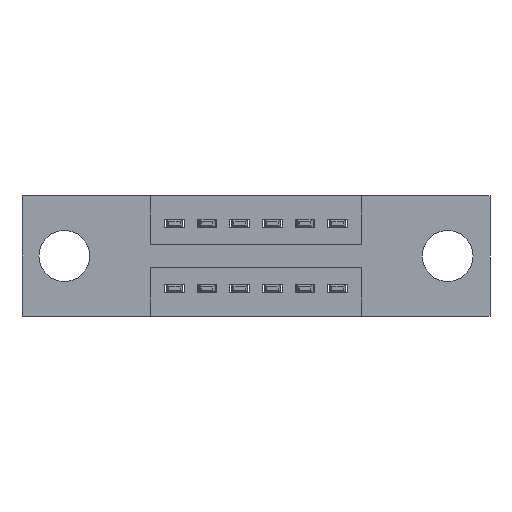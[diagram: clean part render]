
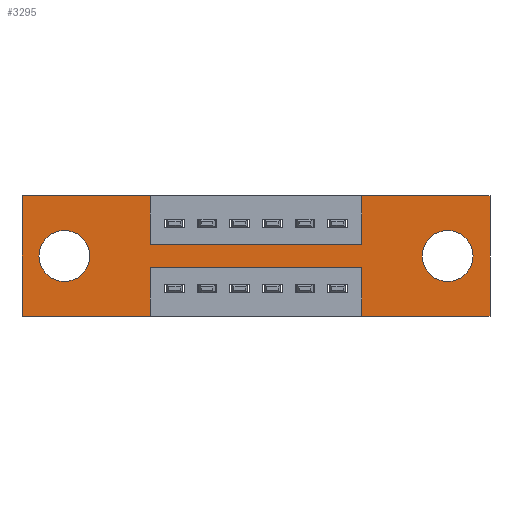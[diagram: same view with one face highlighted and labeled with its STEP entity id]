
A CAD part, front view. The second image highlights one B-rep face of the part: STEP entity #3295.
In plain terms, the highlighted planar face has unit normal (0, -1, 0).
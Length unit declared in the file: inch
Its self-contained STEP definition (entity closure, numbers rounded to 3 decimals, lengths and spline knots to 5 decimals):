
#187 = DIRECTION ( 'NONE',  ( -1., 0., 0. ) ) ;
#217 = VERTEX_POINT ( 'NONE', #2972 ) ;
#337 = LINE ( 'NONE', #4971, #4850 ) ;
#415 = EDGE_CURVE ( 'NONE', #9614, #4297, #8648, .T. ) ;
#434 = ORIENTED_EDGE ( 'NONE', *, *, #8055, .F. ) ;
#477 = CARTESIAN_POINT ( 'NONE',  ( 0.3925, 0., -0.37 ) ) ;
#515 = ORIENTED_EDGE ( 'NONE', *, *, #3587, .F. ) ;
#593 = DIRECTION ( 'NONE',  ( 0., 0., 1. ) ) ;
#698 = EDGE_CURVE ( 'NONE', #9111, #2674, #3773, .T. ) ;
#855 = DIRECTION ( 'NONE',  ( 0., 1., 0. ) ) ;
#882 = EDGE_CURVE ( 'NONE', #5985, #5519, #2591, .T. ) ;
#930 = CARTESIAN_POINT ( 'NONE',  ( 1.435, 0., -0.37 ) ) ;
#1006 = DIRECTION ( 'NONE',  ( 0., 1., 0. ) ) ;
#1039 = CARTESIAN_POINT ( 'NONE',  ( 1.0425, 0., -0.15 ) ) ;
#1098 = DIRECTION ( 'NONE',  ( 0., 0., 1. ) ) ;
#1200 = FACE_OUTER_BOUND ( 'NONE', #3306, .T. ) ;
#1219 = ORIENTED_EDGE ( 'NONE', *, *, #3712, .F. ) ;
#1236 = LINE ( 'NONE', #3494, #9543 ) ;
#1238 = DIRECTION ( 'NONE',  ( 0., 1., 0. ) ) ;
#1439 = EDGE_CURVE ( 'NONE', #4119, #7483, #1813, .T. ) ;
#1510 = CARTESIAN_POINT ( 'NONE',  ( 0., 0., 0. ) ) ;
#1564 = DIRECTION ( 'NONE',  ( -1., 0., 0. ) ) ;
#1686 = ORIENTED_EDGE ( 'NONE', *, *, #415, .T. ) ;
#1782 = VERTEX_POINT ( 'NONE', #6910 ) ;
#1813 = LINE ( 'NONE', #9343, #3753 ) ;
#1977 = VECTOR ( 'NONE', #4465, 39.37008 ) ;
#1980 = CARTESIAN_POINT ( 'NONE',  ( 0.13, 0., -0.185 ) ) ;
#2025 = LINE ( 'NONE', #477, #1977 ) ;
#2029 = DIRECTION ( 'NONE',  ( -1., 0., 0. ) ) ;
#2212 = LINE ( 'NONE', #5299, #7685 ) ;
#2216 = ORIENTED_EDGE ( 'NONE', *, *, #882, .F. ) ;
#2288 = CARTESIAN_POINT ( 'NONE',  ( 1.0425, 0., 0. ) ) ;
#2332 = CARTESIAN_POINT ( 'NONE',  ( 0.13, 0., -0.263 ) ) ;
#2591 = LINE ( 'NONE', #9475, #3455 ) ;
#2674 = VERTEX_POINT ( 'NONE', #2332 ) ;
#2708 = CARTESIAN_POINT ( 'NONE',  ( 1.305, 0., -0.107 ) ) ;
#2804 = AXIS2_PLACEMENT_3D ( 'NONE', #5584, #1006, #4055 ) ;
#2819 = ORIENTED_EDGE ( 'NONE', *, *, #8117, .T. ) ;
#2972 = CARTESIAN_POINT ( 'NONE',  ( 0.3925, 0., -0.22 ) ) ;
#3007 = DIRECTION ( 'NONE',  ( 0., 0., 1. ) ) ;
#3103 = LINE ( 'NONE', #6804, #7696 ) ;
#3113 = EDGE_CURVE ( 'NONE', #7722, #5985, #5393, .T. ) ;
#3295 = ADVANCED_FACE ( 'NONE', ( #8737, #4986, #1200 ), #3510, .T. ) ;
#3306 = EDGE_LOOP ( 'NONE', ( #434, #1219, #2216, #4464, #7397, #6076, #3683, #5480, #3716, #4623, #3730, #515 ) ) ;
#3455 = VECTOR ( 'NONE', #1098, 39.37008 ) ;
#3494 = CARTESIAN_POINT ( 'NONE',  ( 0., 0., 0. ) ) ;
#3510 = PLANE ( 'NONE',  #7396 ) ;
#3587 = EDGE_CURVE ( 'NONE', #8382, #5559, #3103, .T. ) ;
#3589 = EDGE_CURVE ( 'NONE', #7483, #3890, #8487, .T. ) ;
#3603 = VECTOR ( 'NONE', #6065, 39.37008 ) ;
#3683 = ORIENTED_EDGE ( 'NONE', *, *, #3589, .F. ) ;
#3712 = EDGE_CURVE ( 'NONE', #5519, #217, #337, .T. ) ;
#3716 = ORIENTED_EDGE ( 'NONE', *, *, #4641, .F. ) ;
#3730 = ORIENTED_EDGE ( 'NONE', *, *, #4853, .F. ) ;
#3753 = VECTOR ( 'NONE', #4156, 39.37008 ) ;
#3773 = CIRCLE ( 'NONE', #3926, 0.078 ) ;
#3821 = EDGE_LOOP ( 'NONE', ( #1686, #2819 ) ) ;
#3890 = VERTEX_POINT ( 'NONE', #6530 ) ;
#3908 = DIRECTION ( 'NONE',  ( 0., 0., 1. ) ) ;
#3926 = AXIS2_PLACEMENT_3D ( 'NONE', #6165, #855, #3908 ) ;
#4055 = DIRECTION ( 'NONE',  ( 0., 0., -1. ) ) ;
#4119 = VERTEX_POINT ( 'NONE', #4124 ) ;
#4124 = CARTESIAN_POINT ( 'NONE',  ( 0.3925, 0., -0.15 ) ) ;
#4156 = DIRECTION ( 'NONE',  ( 1., 0., 0. ) ) ;
#4297 = VERTEX_POINT ( 'NONE', #5846 ) ;
#4464 = ORIENTED_EDGE ( 'NONE', *, *, #3113, .F. ) ;
#4465 = DIRECTION ( 'NONE',  ( 0., 0., -1. ) ) ;
#4581 = CARTESIAN_POINT ( 'NONE',  ( 0., 0., 0. ) ) ;
#4623 = ORIENTED_EDGE ( 'NONE', *, *, #6403, .F. ) ;
#4641 = EDGE_CURVE ( 'NONE', #1782, #4119, #7011, .T. ) ;
#4748 = CARTESIAN_POINT ( 'NONE',  ( 0., 0., -0.37 ) ) ;
#4850 = VECTOR ( 'NONE', #187, 39.37008 ) ;
#4853 = EDGE_CURVE ( 'NONE', #5559, #5003, #6122, .T. ) ;
#4886 = CARTESIAN_POINT ( 'NONE',  ( 1.435, 0., 0. ) ) ;
#4971 = CARTESIAN_POINT ( 'NONE',  ( 0.3925, 0., -0.22 ) ) ;
#4986 = FACE_BOUND ( 'NONE', #7451, .T. ) ;
#5003 = VERTEX_POINT ( 'NONE', #9190 ) ;
#5151 = CARTESIAN_POINT ( 'NONE',  ( 1.305, 0., -0.185 ) ) ;
#5214 = ORIENTED_EDGE ( 'NONE', *, *, #698, .T. ) ;
#5299 = CARTESIAN_POINT ( 'NONE',  ( 1.435, 0., 0. ) ) ;
#5393 = LINE ( 'NONE', #4748, #9753 ) ;
#5480 = ORIENTED_EDGE ( 'NONE', *, *, #1439, .F. ) ;
#5519 = VERTEX_POINT ( 'NONE', #6654 ) ;
#5537 = DIRECTION ( 'NONE',  ( 0., -1., 0. ) ) ;
#5559 = VERTEX_POINT ( 'NONE', #8893 ) ;
#5584 = CARTESIAN_POINT ( 'NONE',  ( 1.305, 0., -0.185 ) ) ;
#5640 = DIRECTION ( 'NONE',  ( 0., 0., -1. ) ) ;
#5846 = CARTESIAN_POINT ( 'NONE',  ( 1.305, 0., -0.263 ) ) ;
#5889 = DIRECTION ( 'NONE',  ( 1., 0., 0. ) ) ;
#5985 = VERTEX_POINT ( 'NONE', #8044 ) ;
#6065 = DIRECTION ( 'NONE',  ( 0., 0., 1. ) ) ;
#6076 = ORIENTED_EDGE ( 'NONE', *, *, #7782, .F. ) ;
#6087 = LINE ( 'NONE', #4581, #9257 ) ;
#6122 = LINE ( 'NONE', #1510, #3603 ) ;
#6165 = CARTESIAN_POINT ( 'NONE',  ( 0.13, 0., -0.185 ) ) ;
#6403 = EDGE_CURVE ( 'NONE', #5003, #1782, #1236, .T. ) ;
#6477 = DIRECTION ( 'NONE',  ( 0., 1., 0. ) ) ;
#6501 = CARTESIAN_POINT ( 'NONE',  ( 0., 0., -0.37 ) ) ;
#6530 = CARTESIAN_POINT ( 'NONE',  ( 1.0425, 0., 0. ) ) ;
#6602 = DIRECTION ( 'NONE',  ( 0., 0., -1. ) ) ;
#6654 = CARTESIAN_POINT ( 'NONE',  ( 1.0425, 0., -0.22 ) ) ;
#6714 = AXIS2_PLACEMENT_3D ( 'NONE', #1980, #1238, #593 ) ;
#6804 = CARTESIAN_POINT ( 'NONE',  ( 0., 0., -0.37 ) ) ;
#6874 = CIRCLE ( 'NONE', #6714, 0.078 ) ;
#6910 = CARTESIAN_POINT ( 'NONE',  ( 0.3925, 0., 0. ) ) ;
#7011 = LINE ( 'NONE', #7071, #7881 ) ;
#7071 = CARTESIAN_POINT ( 'NONE',  ( 0.3925, 0., 0. ) ) ;
#7317 = ORIENTED_EDGE ( 'NONE', *, *, #7580, .T. ) ;
#7373 = DIRECTION ( 'NONE',  ( 0., 0., -1. ) ) ;
#7396 = AXIS2_PLACEMENT_3D ( 'NONE', #6501, #5537, #6602 ) ;
#7397 = ORIENTED_EDGE ( 'NONE', *, *, #8190, .F. ) ;
#7411 = VERTEX_POINT ( 'NONE', #4886 ) ;
#7451 = EDGE_LOOP ( 'NONE', ( #5214, #7317 ) ) ;
#7483 = VERTEX_POINT ( 'NONE', #1039 ) ;
#7520 = DIRECTION ( 'NONE',  ( 0., 0., -1. ) ) ;
#7580 = EDGE_CURVE ( 'NONE', #2674, #9111, #6874, .T. ) ;
#7684 = DIRECTION ( 'NONE',  ( 1., 0., 0. ) ) ;
#7685 = VECTOR ( 'NONE', #7520, 39.37008 ) ;
#7696 = VECTOR ( 'NONE', #2029, 39.37008 ) ;
#7722 = VERTEX_POINT ( 'NONE', #930 ) ;
#7782 = EDGE_CURVE ( 'NONE', #3890, #7411, #6087, .T. ) ;
#7810 = CARTESIAN_POINT ( 'NONE',  ( 0.3925, 0., -0.37 ) ) ;
#7881 = VECTOR ( 'NONE', #5640, 39.37008 ) ;
#8044 = CARTESIAN_POINT ( 'NONE',  ( 1.0425, 0., -0.37 ) ) ;
#8055 = EDGE_CURVE ( 'NONE', #217, #8382, #2025, .T. ) ;
#8117 = EDGE_CURVE ( 'NONE', #4297, #9614, #9412, .T. ) ;
#8190 = EDGE_CURVE ( 'NONE', #7411, #7722, #2212, .T. ) ;
#8316 = AXIS2_PLACEMENT_3D ( 'NONE', #5151, #6477, #7373 ) ;
#8382 = VERTEX_POINT ( 'NONE', #7810 ) ;
#8487 = LINE ( 'NONE', #2288, #9103 ) ;
#8648 = CIRCLE ( 'NONE', #2804, 0.078 ) ;
#8737 = FACE_BOUND ( 'NONE', #3821, .T. ) ;
#8893 = CARTESIAN_POINT ( 'NONE',  ( 0., 0., -0.37 ) ) ;
#9103 = VECTOR ( 'NONE', #3007, 39.37008 ) ;
#9111 = VERTEX_POINT ( 'NONE', #9114 ) ;
#9114 = CARTESIAN_POINT ( 'NONE',  ( 0.13, 0., -0.107 ) ) ;
#9190 = CARTESIAN_POINT ( 'NONE',  ( 0., 0., 0. ) ) ;
#9257 = VECTOR ( 'NONE', #7684, 39.37008 ) ;
#9343 = CARTESIAN_POINT ( 'NONE',  ( 0.3925, 0., -0.15 ) ) ;
#9412 = CIRCLE ( 'NONE', #8316, 0.078 ) ;
#9475 = CARTESIAN_POINT ( 'NONE',  ( 1.0425, 0., -0.37 ) ) ;
#9543 = VECTOR ( 'NONE', #5889, 39.37008 ) ;
#9614 = VERTEX_POINT ( 'NONE', #2708 ) ;
#9753 = VECTOR ( 'NONE', #1564, 39.37008 ) ;
